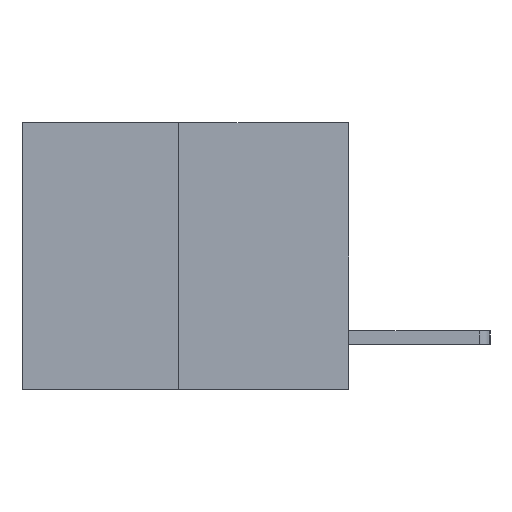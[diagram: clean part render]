
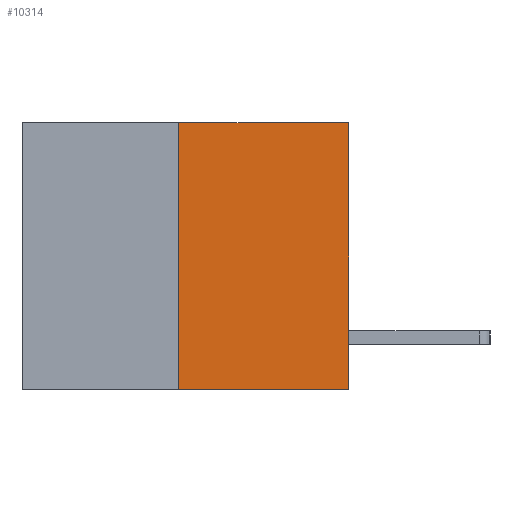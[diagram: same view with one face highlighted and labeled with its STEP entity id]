
A CAD part, left-side view. The second image highlights one B-rep face of the part: STEP entity #10314.
In plain terms, the highlighted planar face has unit normal (-1, 0, 0).
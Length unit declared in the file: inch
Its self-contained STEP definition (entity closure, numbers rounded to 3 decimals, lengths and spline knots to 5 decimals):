
#237 = ORIENTED_EDGE ( 'NONE', *, *, #6549, .F. ) ;
#286 = CARTESIAN_POINT ( 'NONE',  ( 0., 0.312, -0.49 ) ) ;
#386 = CARTESIAN_POINT ( 'NONE',  ( 0., 0.312, 0. ) ) ;
#497 = CARTESIAN_POINT ( 'NONE',  ( 0., 0.312, -0.49 ) ) ;
#576 = CARTESIAN_POINT ( 'NONE',  ( 0., 0.6, 0. ) ) ;
#1387 = DIRECTION ( 'NONE',  ( 0., -1., 0. ) ) ;
#1470 = VERTEX_POINT ( 'NONE', #10842 ) ;
#2953 = AXIS2_PLACEMENT_3D ( 'NONE', #2954, #6242, #7089 ) ;
#2954 = CARTESIAN_POINT ( 'NONE',  ( 0., 0.6, 0. ) ) ;
#3339 = VECTOR ( 'NONE', #9628, 39.37008 ) ;
#3722 = EDGE_CURVE ( 'NONE', #10888, #1470, #5824, .T. ) ;
#3907 = DIRECTION ( 'NONE',  ( 0., -1., 0. ) ) ;
#4223 = FACE_OUTER_BOUND ( 'NONE', #5890, .T. ) ;
#4359 = EDGE_CURVE ( 'NONE', #5424, #1470, #9615, .T. ) ;
#5240 = CARTESIAN_POINT ( 'NONE',  ( 0., 0., -0.49 ) ) ;
#5424 = VERTEX_POINT ( 'NONE', #386 ) ;
#5824 = LINE ( 'NONE', #6985, #3339 ) ;
#5890 = EDGE_LOOP ( 'NONE', ( #237, #5930, #10491, #8348 ) ) ;
#5930 = ORIENTED_EDGE ( 'NONE', *, *, #10500, .T. ) ;
#6242 = DIRECTION ( 'NONE',  ( 1., 0., 0. ) ) ;
#6334 = VECTOR ( 'NONE', #1387, 39.37008 ) ;
#6436 = VECTOR ( 'NONE', #3907, 39.37008 ) ;
#6549 = EDGE_CURVE ( 'NONE', #9806, #5424, #8503, .T. ) ;
#6562 = LINE ( 'NONE', #10577, #6436 ) ;
#6985 = CARTESIAN_POINT ( 'NONE',  ( 0., 0., 0. ) ) ;
#7089 = DIRECTION ( 'NONE',  ( 0., 0., -1. ) ) ;
#7158 = PLANE ( 'NONE',  #2953 ) ;
#8348 = ORIENTED_EDGE ( 'NONE', *, *, #4359, .F. ) ;
#8503 = LINE ( 'NONE', #286, #9941 ) ;
#9615 = LINE ( 'NONE', #576, #6334 ) ;
#9628 = DIRECTION ( 'NONE',  ( 0., 0., 1. ) ) ;
#9806 = VERTEX_POINT ( 'NONE', #497 ) ;
#9941 = VECTOR ( 'NONE', #10501, 39.37008 ) ;
#10314 = ADVANCED_FACE ( 'NONE', ( #4223 ), #7158, .F. ) ;
#10491 = ORIENTED_EDGE ( 'NONE', *, *, #3722, .T. ) ;
#10500 = EDGE_CURVE ( 'NONE', #9806, #10888, #6562, .T. ) ;
#10501 = DIRECTION ( 'NONE',  ( 0., 0., 1. ) ) ;
#10577 = CARTESIAN_POINT ( 'NONE',  ( 0., 0.6, -0.49 ) ) ;
#10842 = CARTESIAN_POINT ( 'NONE',  ( 0., 0., 0. ) ) ;
#10888 = VERTEX_POINT ( 'NONE', #5240 ) ;
